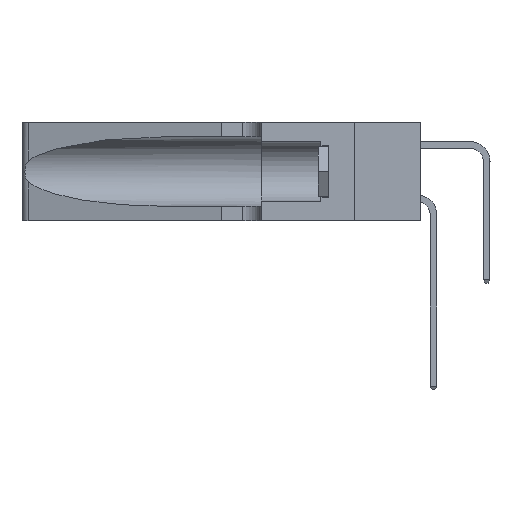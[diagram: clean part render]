
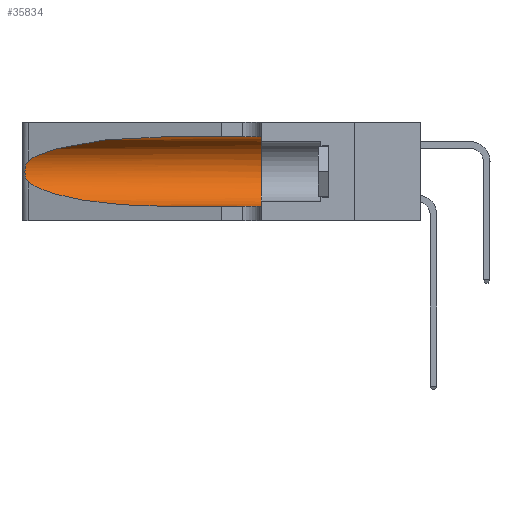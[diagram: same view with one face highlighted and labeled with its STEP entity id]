
A CAD part, left-side view. The second image highlights one B-rep face of the part: STEP entity #35834.
In plain terms, the highlighted cylindrical face has radius 3.308 mm (diameter 6.617 mm), a partial arc.
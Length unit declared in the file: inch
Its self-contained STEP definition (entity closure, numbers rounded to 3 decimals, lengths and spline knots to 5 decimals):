
#578 = CARTESIAN_POINT ( 'NONE',  ( 0.25789, 1.23486, 0.15765 ) ) ;
#2357 = VERTEX_POINT ( 'NONE', #26692 ) ;
#2867 = B_SPLINE_CURVE_WITH_KNOTS ( 'NONE', 3,
 ( #4200, #25822, #32921, #11575, #36496, #15230, #40041, #18832, #43627, #22416, #578, #25975, #4364, #29532 ),
 .UNSPECIFIED., .F., .F.,
 ( 4, 2, 2, 2, 2, 2, 4 ),
 ( 0., 0.00027, 0.00053, 0.00107, 0.0016, 0.00187, 0.00214 ),
 .UNSPECIFIED. ) ;
#3018 = EDGE_CURVE ( 'NONE', #20677, #12702, #9143, .T. ) ;
#4200 = CARTESIAN_POINT ( 'NONE',  ( 0.25487, 1.22718, 0.22369 ) ) ;
#4364 = CARTESIAN_POINT ( 'NONE',  ( 0.25555, 1.22993, 0.14849 ) ) ;
#4881 = CARTESIAN_POINT ( 'NONE',  ( 0.1305, 1.61858, 0.31525 ) ) ;
#8370 = DIRECTION ( 'NONE',  ( 0., 1., 0. ) ) ;
#9143 = LINE ( 'NONE', #4881, #37613 ) ;
#9833 = VECTOR ( 'NONE', #40210, 39.37008 ) ;
#10040 = VERTEX_POINT ( 'NONE', #46524 ) ;
#11575 = CARTESIAN_POINT ( 'NONE',  ( 0.25787, 1.23484, 0.2124 ) ) ;
#12702 = VERTEX_POINT ( 'NONE', #33307 ) ;
#12993 = CARTESIAN_POINT ( 'NONE',  ( 0.25487, 1.22718, 0.22369 ) ) ;
#14122 = VERTEX_POINT ( 'NONE', #40627 ) ;
#14517 = CARTESIAN_POINT ( 'NONE',  ( 0.1305, 0.72297, 0.05475 ) ) ;
#14643 = CARTESIAN_POINT ( 'NONE',  ( 0.25487, 1.22718, 0.22369 ) ) ;
#15134 = CARTESIAN_POINT ( 'NONE',  ( 0.1305, 0.72297, 0.31525 ) ) ;
#15230 = CARTESIAN_POINT ( 'NONE',  ( 0.26018, 1.23835, 0.19895 ) ) ;
#15399 = CARTESIAN_POINT ( 'NONE',  ( 0.1305, 1.61858, 0.05475 ) ) ;
#18057 = DIRECTION ( 'NONE',  ( 0., -1., 0. ) ) ;
#18095 = ORIENTED_EDGE ( 'NONE', *, *, #46003, .T. ) ;
#18373 = DIRECTION ( 'NONE',  ( 0., 0., -1. ) ) ;
#18832 = CARTESIAN_POINT ( 'NONE',  ( 0.26075, 1.23896, 0.178 ) ) ;
#20649 = EDGE_LOOP ( 'NONE', ( #34688, #34354, #18095, #21875, #39044, #25553 ) ) ;
#20677 = VERTEX_POINT ( 'NONE', #15134 ) ;
#21222 =( BOUNDED_CURVE ( )  B_SPLINE_CURVE ( 3, ( #32231, #46358, #35809, #14517 ),
 .UNSPECIFIED., .F., .T. ) 
 B_SPLINE_CURVE_WITH_KNOTS ( ( 4, 4 ),
 ( 3.44316, 4.71239 ),
 .UNSPECIFIED. ) 
 CURVE ( )  GEOMETRIC_REPRESENTATION_ITEM ( )  RATIONAL_B_SPLINE_CURVE ( ( 1., 0.87, 0.87, 1. ) ) 
 REPRESENTATION_ITEM ( '' )  );
#21875 = ORIENTED_EDGE ( 'NONE', *, *, #44537, .T. ) ;
#22416 = CARTESIAN_POINT ( 'NONE',  ( 0.25856, 1.23593, 0.16098 ) ) ;
#25508 = CARTESIAN_POINT ( 'NONE',  ( 0.1305, 1.61858, 0.185 ) ) ;
#25553 = ORIENTED_EDGE ( 'NONE', *, *, #3018, .F. ) ;
#25822 = CARTESIAN_POINT ( 'NONE',  ( 0.25555, 1.22994, 0.2215 ) ) ;
#25975 = CARTESIAN_POINT ( 'NONE',  ( 0.25639, 1.23186, 0.15144 ) ) ;
#26484 = DIRECTION ( 'NONE',  ( 0., -1., 0. ) ) ;
#26692 = CARTESIAN_POINT ( 'NONE',  ( 0.1305, 0.72297, 0.05475 ) ) ;
#27029 = EDGE_CURVE ( 'NONE', #31291, #14122, #2867, .T. ) ;
#27206 = CARTESIAN_POINT ( 'NONE',  ( 0.1305, 0.72297, 0.31525 ) ) ;
#27257 = EDGE_CURVE ( 'NONE', #20677, #31291, #41101, .T. ) ;
#29532 = CARTESIAN_POINT ( 'NONE',  ( 0.25487, 1.22718, 0.14631 ) ) ;
#29819 = CARTESIAN_POINT ( 'NONE',  ( 0.1305, 0.35, 0.185 ) ) ;
#31291 = VERTEX_POINT ( 'NONE', #14643 ) ;
#32114 = EDGE_CURVE ( 'NONE', #12702, #10040, #40839, .T. ) ;
#32231 = CARTESIAN_POINT ( 'NONE',  ( 0.25487, 1.22718, 0.14631 ) ) ;
#32921 = CARTESIAN_POINT ( 'NONE',  ( 0.25639, 1.23184, 0.21858 ) ) ;
#33307 = CARTESIAN_POINT ( 'NONE',  ( 0.1305, 0.35, 0.31525 ) ) ;
#33376 = DIRECTION ( 'NONE',  ( 0., 0., 1. ) ) ;
#34308 = CARTESIAN_POINT ( 'NONE',  ( 0.2373, 1.15595, 0.28018 ) ) ;
#34354 = ORIENTED_EDGE ( 'NONE', *, *, #27029, .T. ) ;
#34688 = ORIENTED_EDGE ( 'NONE', *, *, #27257, .T. ) ;
#35809 = CARTESIAN_POINT ( 'NONE',  ( 0.18966, 0.96281, 0.05475 ) ) ;
#35834 = ADVANCED_FACE ( 'NONE', ( #36690 ), #45020, .F. ) ;
#36086 = LINE ( 'NONE', #15399, #9833 ) ;
#36496 = CARTESIAN_POINT ( 'NONE',  ( 0.25854, 1.2359, 0.20912 ) ) ;
#36690 = FACE_OUTER_BOUND ( 'NONE', #20649, .T. ) ;
#37613 = VECTOR ( 'NONE', #26484, 39.37008 ) ;
#39044 = ORIENTED_EDGE ( 'NONE', *, *, #32114, .F. ) ;
#40041 = CARTESIAN_POINT ( 'NONE',  ( 0.26075, 1.23896, 0.19203 ) ) ;
#40210 = DIRECTION ( 'NONE',  ( 0., -1., 0. ) ) ;
#40627 = CARTESIAN_POINT ( 'NONE',  ( 0.25487, 1.22718, 0.14631 ) ) ;
#40839 = CIRCLE ( 'NONE', #43594, 0.13025 ) ;
#41101 =( BOUNDED_CURVE ( )  B_SPLINE_CURVE ( 3, ( #27206, #44855, #34308, #12993 ),
 .UNSPECIFIED., .F., .T. ) 
 B_SPLINE_CURVE_WITH_KNOTS ( ( 4, 4 ),
 ( 1.5708, 2.84003 ),
 .UNSPECIFIED. ) 
 CURVE ( )  GEOMETRIC_REPRESENTATION_ITEM ( )  RATIONAL_B_SPLINE_CURVE ( ( 1., 0.87, 0.87, 1. ) ) 
 REPRESENTATION_ITEM ( '' )  );
#42486 = AXIS2_PLACEMENT_3D ( 'NONE', #25508, #18057, #18373 ) ;
#43594 = AXIS2_PLACEMENT_3D ( 'NONE', #29819, #8370, #33376 ) ;
#43627 = CARTESIAN_POINT ( 'NONE',  ( 0.26017, 1.23833, 0.17102 ) ) ;
#44537 = EDGE_CURVE ( 'NONE', #2357, #10040, #36086, .T. ) ;
#44855 = CARTESIAN_POINT ( 'NONE',  ( 0.18966, 0.96281, 0.31525 ) ) ;
#45020 = CYLINDRICAL_SURFACE ( 'NONE', #42486, 0.13025 ) ;
#46003 = EDGE_CURVE ( 'NONE', #14122, #2357, #21222, .T. ) ;
#46358 = CARTESIAN_POINT ( 'NONE',  ( 0.2373, 1.15595, 0.08982 ) ) ;
#46524 = CARTESIAN_POINT ( 'NONE',  ( 0.1305, 0.35, 0.05475 ) ) ;
